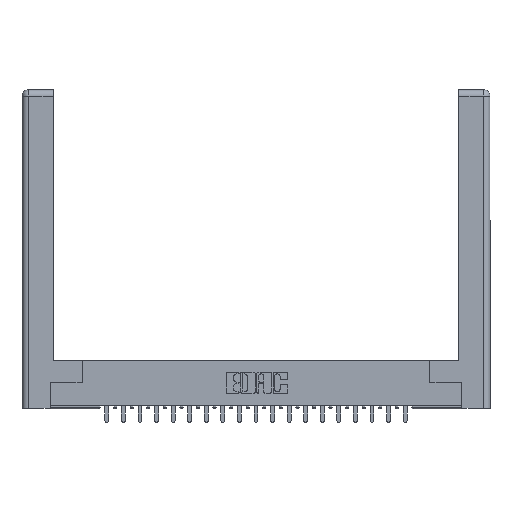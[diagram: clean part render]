
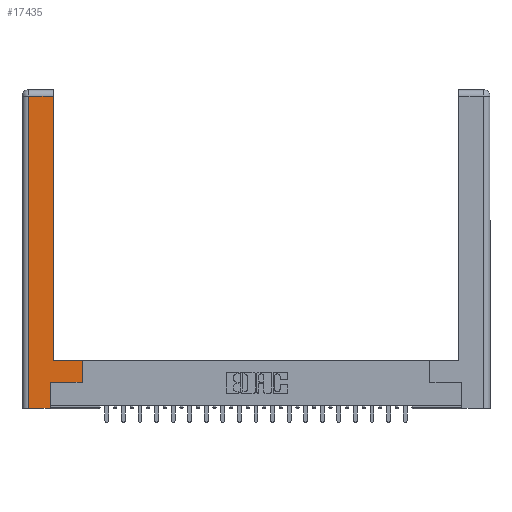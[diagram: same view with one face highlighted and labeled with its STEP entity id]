
A CAD part, top view. The second image highlights one B-rep face of the part: STEP entity #17435.
In plain terms, the highlighted planar face has unit normal (0, 0, 1).
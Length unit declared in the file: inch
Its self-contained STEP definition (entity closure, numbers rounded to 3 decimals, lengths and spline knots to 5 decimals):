
#71 = CARTESIAN_POINT ( 'NONE',  ( 0., 0., 0. ) ) ;
#271 = VECTOR ( 'NONE', #10276, 39.37008 ) ;
#329 = DIRECTION ( 'NONE',  ( 0., 1., 0. ) ) ;
#819 = VERTEX_POINT ( 'NONE', #23215 ) ;
#979 = EDGE_CURVE ( 'NONE', #17205, #819, #22351, .T. ) ;
#1137 = CARTESIAN_POINT ( 'NONE',  ( 0.565, 0.245, 0. ) ) ;
#1418 = DIRECTION ( 'NONE',  ( 1., 0., 0. ) ) ;
#1901 = DIRECTION ( 'NONE',  ( -1., 0., 0. ) ) ;
#1944 = LINE ( 'NONE', #11221, #12153 ) ;
#1960 = AXIS2_PLACEMENT_3D ( 'NONE', #71, #12751, #1901 ) ;
#2034 = ORIENTED_EDGE ( 'NONE', *, *, #3065, .T. ) ;
#3065 = EDGE_CURVE ( 'NONE', #11944, #14394, #21986, .T. ) ;
#3327 = CARTESIAN_POINT ( 'NONE',  ( 0.565, 0.245, 0. ) ) ;
#3838 = CARTESIAN_POINT ( 'NONE',  ( 0.295, 2.94, 0. ) ) ;
#4783 = CARTESIAN_POINT ( 'NONE',  ( 0.565, 0.45, 0. ) ) ;
#5120 = LINE ( 'NONE', #1137, #271 ) ;
#5132 = VECTOR ( 'NONE', #20147, 39.37008 ) ;
#5290 = VERTEX_POINT ( 'NONE', #8004 ) ;
#5348 = EDGE_CURVE ( 'NONE', #5290, #5887, #13913, .T. ) ;
#5711 = ORIENTED_EDGE ( 'NONE', *, *, #14146, .T. ) ;
#5887 = VERTEX_POINT ( 'NONE', #9607 ) ;
#7200 = DIRECTION ( 'NONE',  ( -1., 0., 0. ) ) ;
#7263 = CARTESIAN_POINT ( 'NONE',  ( 0.295, 0.45, 0. ) ) ;
#7475 = CARTESIAN_POINT ( 'NONE',  ( 0.0615, 2.94, 0. ) ) ;
#7585 = ORIENTED_EDGE ( 'NONE', *, *, #16097, .T. ) ;
#7603 = CARTESIAN_POINT ( 'NONE',  ( 0.0615, 2.94, 0. ) ) ;
#7907 = VECTOR ( 'NONE', #1418, 39.37008 ) ;
#8004 = CARTESIAN_POINT ( 'NONE',  ( 0.265, 0., 0. ) ) ;
#8086 = CARTESIAN_POINT ( 'NONE',  ( 0.265, 0.245, 0. ) ) ;
#9154 = VECTOR ( 'NONE', #22398, 39.37008 ) ;
#9607 = CARTESIAN_POINT ( 'NONE',  ( 0.265, 0.245, 0. ) ) ;
#10276 = DIRECTION ( 'NONE',  ( 1., 0., 0. ) ) ;
#10448 = DIRECTION ( 'NONE',  ( 0., -1., 0. ) ) ;
#10505 = EDGE_CURVE ( 'NONE', #819, #11944, #22197, .T. ) ;
#11035 = ORIENTED_EDGE ( 'NONE', *, *, #10505, .T. ) ;
#11221 = CARTESIAN_POINT ( 'NONE',  ( 0.565, 0.45, 0. ) ) ;
#11841 = ORIENTED_EDGE ( 'NONE', *, *, #5348, .T. ) ;
#11944 = VERTEX_POINT ( 'NONE', #3838 ) ;
#12153 = VECTOR ( 'NONE', #329, 39.37008 ) ;
#12432 = VERTEX_POINT ( 'NONE', #3327 ) ;
#12751 = DIRECTION ( 'NONE',  ( 0., 0., -1. ) ) ;
#12790 = LINE ( 'NONE', #22866, #13346 ) ;
#13346 = VECTOR ( 'NONE', #10448, 39.37008 ) ;
#13913 = LINE ( 'NONE', #8086, #9154 ) ;
#14146 = EDGE_CURVE ( 'NONE', #14394, #21298, #12790, .T. ) ;
#14394 = VERTEX_POINT ( 'NONE', #7475 ) ;
#15235 = FACE_OUTER_BOUND ( 'NONE', #20948, .T. ) ;
#15839 = CARTESIAN_POINT ( 'NONE',  ( 0.295, 3., 0. ) ) ;
#15908 = CARTESIAN_POINT ( 'NONE',  ( 0.265, 0., 0. ) ) ;
#16097 = EDGE_CURVE ( 'NONE', #5887, #12432, #5120, .T. ) ;
#16193 = ORIENTED_EDGE ( 'NONE', *, *, #17311, .T. ) ;
#16301 = PLANE ( 'NONE',  #1960 ) ;
#16947 = EDGE_CURVE ( 'NONE', #12432, #17205, #1944, .T. ) ;
#17205 = VERTEX_POINT ( 'NONE', #4783 ) ;
#17311 = EDGE_CURVE ( 'NONE', #21298, #5290, #17465, .T. ) ;
#17435 = ADVANCED_FACE ( 'NONE', ( #15235 ), #16301, .F. ) ;
#17465 = LINE ( 'NONE', #15908, #7907 ) ;
#17628 = DIRECTION ( 'NONE',  ( 0., 1., 0. ) ) ;
#18231 = ORIENTED_EDGE ( 'NONE', *, *, #16947, .T. ) ;
#18675 = CARTESIAN_POINT ( 'NONE',  ( 0.0615, 0., 0. ) ) ;
#20081 = ORIENTED_EDGE ( 'NONE', *, *, #979, .T. ) ;
#20147 = DIRECTION ( 'NONE',  ( -1., 0., 0. ) ) ;
#20536 = VECTOR ( 'NONE', #17628, 39.37008 ) ;
#20948 = EDGE_LOOP ( 'NONE', ( #11035, #2034, #5711, #16193, #11841, #7585, #18231, #20081 ) ) ;
#21298 = VERTEX_POINT ( 'NONE', #18675 ) ;
#21986 = LINE ( 'NONE', #7603, #5132 ) ;
#22197 = LINE ( 'NONE', #15839, #20536 ) ;
#22351 = LINE ( 'NONE', #7263, #22886 ) ;
#22398 = DIRECTION ( 'NONE',  ( 0., 1., 0. ) ) ;
#22866 = CARTESIAN_POINT ( 'NONE',  ( 0.0615, 0., 0. ) ) ;
#22886 = VECTOR ( 'NONE', #7200, 39.37008 ) ;
#23215 = CARTESIAN_POINT ( 'NONE',  ( 0.295, 0.45, 0. ) ) ;
